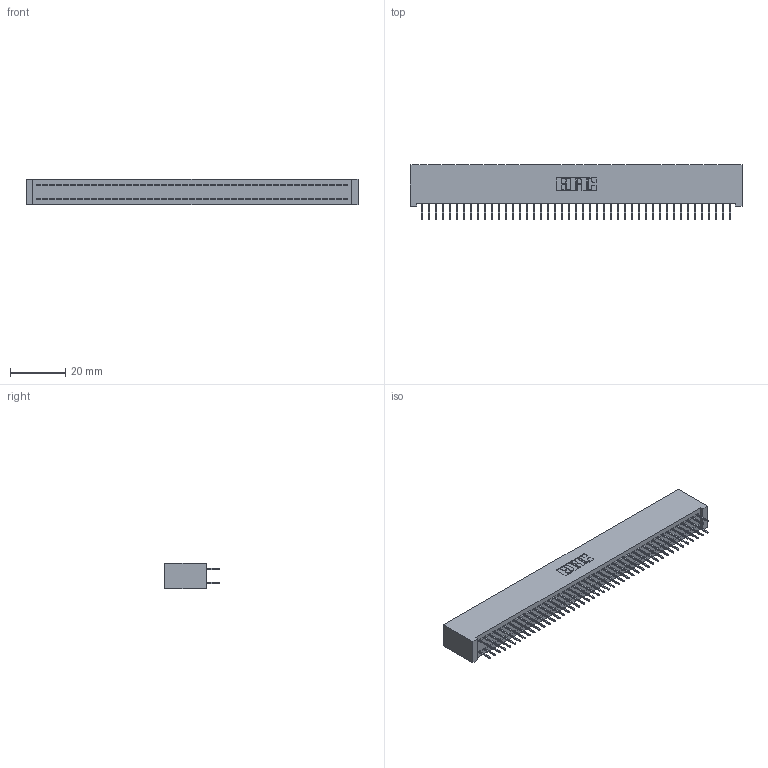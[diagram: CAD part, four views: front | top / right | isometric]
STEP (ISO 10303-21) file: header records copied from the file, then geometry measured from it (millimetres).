
FILE_DESCRIPTION (( 'STEP AP203' ), '1' );
FILE_NAME ('392-090-524-201.STEP', '2018-08-18T06:54:16', ( '' ), ( '' ), 'SwSTEP 2.0', 'SolidWorks 2016', '' );
FILE_SCHEMA (( 'CONFIG_CONTROL_DESIGN' ));
Length unit declared in the file: inch
Products named in the file (3): 342 Part_Lugless; 345-292-001_345-293-124; 392-090-524-201
Assembly tree (91 placements, depth 2):
  392-090-524-201
    342 Part_Lugless
    345-292-001_345-293-124  x90
Bounding box: 120.55 x 19.69 x 9.4 mm (x, y, z)
Volume: 11148.8 mm3; surface area: 18313.3 mm2
Topology: 91 solids, 91 shells, 5142 faces, 14585 edges, 9362 vertices
Faces by surface type: plane 3842, cylinder 1300
Entity records: 28227 total; most frequent: CARTESIAN_POINT 4670, ORIENTED_EDGE 4606, DIRECTION 3979, EDGE_CURVE 2303, VECTOR 2187, LINE 2187, VERTEX_POINT 1530, AXIS2_PLACEMENT_3D 896
